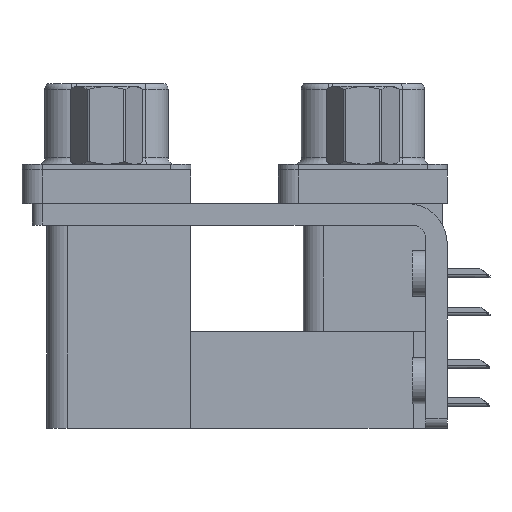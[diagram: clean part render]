
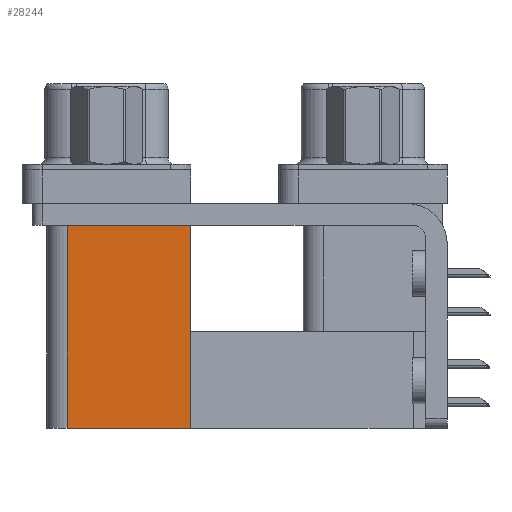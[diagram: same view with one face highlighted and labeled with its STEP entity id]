
A CAD part, left-side view. The second image highlights one B-rep face of the part: STEP entity #28244.
In plain terms, the highlighted planar face has unit normal (-1, 0, 0).
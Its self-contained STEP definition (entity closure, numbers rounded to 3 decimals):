
#1496 = EDGE_CURVE ( 'NONE', #34206, #19539, #29549, .T. ) ;
#1729 = VECTOR ( 'NONE', #35090, 1000. ) ;
#3835 = CARTESIAN_POINT ( 'NONE',  ( 3.765, 12.775, -19.2 ) ) ;
#4261 = LINE ( 'NONE', #7584, #30304 ) ;
#4647 = DIRECTION ( 'NONE',  ( 0., 1., 0. ) ) ;
#6557 = DIRECTION ( 'NONE',  ( 0., 0., -1. ) ) ;
#7584 = CARTESIAN_POINT ( 'NONE',  ( 3.765, 12.775, -2.5 ) ) ;
#8172 = ORIENTED_EDGE ( 'NONE', *, *, #31854, .T. ) ;
#9475 = FACE_OUTER_BOUND ( 'NONE', #23506, .T. ) ;
#11251 = ORIENTED_EDGE ( 'NONE', *, *, #37375, .F. ) ;
#14162 = CARTESIAN_POINT ( 'NONE',  ( 3.765, 21.975, -19.2 ) ) ;
#15533 = PLANE ( 'NONE',  #33363 ) ;
#17107 = DIRECTION ( 'NONE',  ( 0., 0., 1. ) ) ;
#18049 = VERTEX_POINT ( 'NONE', #28970 ) ;
#19539 = VERTEX_POINT ( 'NONE', #37333 ) ;
#21421 = CARTESIAN_POINT ( 'NONE',  ( 3.765, 12.775, -19.2 ) ) ;
#22913 = DIRECTION ( 'NONE',  ( 0., 1., 0. ) ) ;
#23365 = LINE ( 'NONE', #14162, #24797 ) ;
#23506 = EDGE_LOOP ( 'NONE', ( #8172, #11251, #37331, #37657 ) ) ;
#24797 = VECTOR ( 'NONE', #17107, 1000. ) ;
#27018 = VECTOR ( 'NONE', #22913, 1000. ) ;
#28244 = ADVANCED_FACE ( 'NONE', ( #9475 ), #15533, .F. ) ;
#28825 = CARTESIAN_POINT ( 'NONE',  ( 3.765, 12.775, -19.2 ) ) ;
#28970 = CARTESIAN_POINT ( 'NONE',  ( 3.765, 12.775, -2.5 ) ) ;
#29220 = LINE ( 'NONE', #28825, #1729 ) ;
#29549 = LINE ( 'NONE', #31902, #27018 ) ;
#30304 = VECTOR ( 'NONE', #4647, 1000. ) ;
#30540 = VERTEX_POINT ( 'NONE', #30836 ) ;
#30836 = CARTESIAN_POINT ( 'NONE',  ( 3.765, 21.975, -2.5 ) ) ;
#31854 = EDGE_CURVE ( 'NONE', #18049, #30540, #4261, .T. ) ;
#31902 = CARTESIAN_POINT ( 'NONE',  ( 3.765, 12.775, -19.2 ) ) ;
#33332 = DIRECTION ( 'NONE',  ( 1., 0., 0. ) ) ;
#33363 = AXIS2_PLACEMENT_3D ( 'NONE', #21421, #33332, #6557 ) ;
#34206 = VERTEX_POINT ( 'NONE', #3835 ) ;
#34543 = EDGE_CURVE ( 'NONE', #34206, #18049, #29220, .T. ) ;
#35090 = DIRECTION ( 'NONE',  ( 0., 0., 1. ) ) ;
#37331 = ORIENTED_EDGE ( 'NONE', *, *, #1496, .F. ) ;
#37333 = CARTESIAN_POINT ( 'NONE',  ( 3.765, 21.975, -19.2 ) ) ;
#37375 = EDGE_CURVE ( 'NONE', #19539, #30540, #23365, .T. ) ;
#37657 = ORIENTED_EDGE ( 'NONE', *, *, #34543, .T. ) ;
